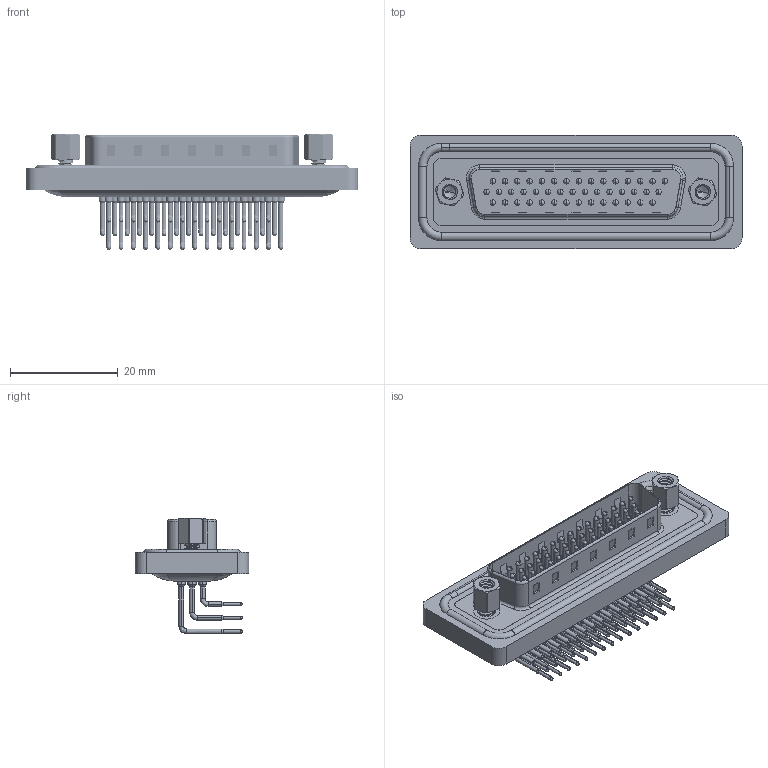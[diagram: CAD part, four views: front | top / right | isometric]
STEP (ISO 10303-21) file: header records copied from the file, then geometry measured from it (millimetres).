
FILE_DESCRIPTION (( 'STEP AP203' ), '1' );
FILE_NAME ('633-W44-362-012.STEP', '2024-04-12T18:35:20', ( '' ), ( '' ), 'SwSTEP 2.0', 'SolidWorks 2023', '' );
FILE_SCHEMA (( 'CONFIG_CONTROL_DESIGN' ));
Length unit declared in the file: millimetre
Products named in the file (9): 633W 4-40 Hex Standoff; 633W Shell_44 Contacts; 633-W44-362-012; 633W Contact Row 2; 633W 4-40 Threaded Rivet_Stabilizer; 633W Waterproof Housing_44 Contacts; 633W Housing_44 Contacts; 633W Contact Row 3; 633W Contact Row 1
Assembly tree (51 placements, depth 2):
  633-W44-362-012
    633W Housing_44 Contacts
    633W Shell_44 Contacts
    633W Waterproof Housing_44 Contacts
    633W Contact Row 1  x15
    633W Contact Row 2  x15
    633W Contact Row 3  x14
    633W 4-40 Threaded Rivet_Stabilizer  x2
    633W 4-40 Hex Standoff  x2
Bounding box: 61.74 x 21.1 x 21.52 mm (x, y, z)
Volume: 6673.6 mm3; surface area: 13580.6 mm2
Topology: 52 solids, 52 shells, 5440 faces, 15264 edges, 9939 vertices
Faces by surface type: plane 3021, cylinder 1886, bspline 286, cone 204, torus 43
Entity records: 42589 total; most frequent: CARTESIAN_POINT 10727, DIRECTION 6489, ORIENTED_EDGE 6002, EDGE_CURVE 3001, AXIS2_PLACEMENT_3D 2438, VERTEX_POINT 1963, LINE 1613, VECTOR 1613
